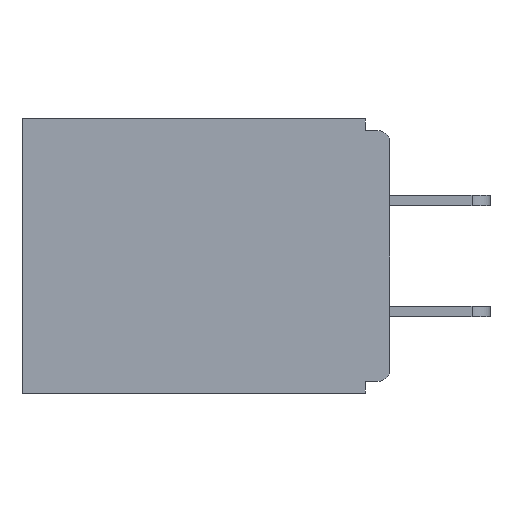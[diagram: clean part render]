
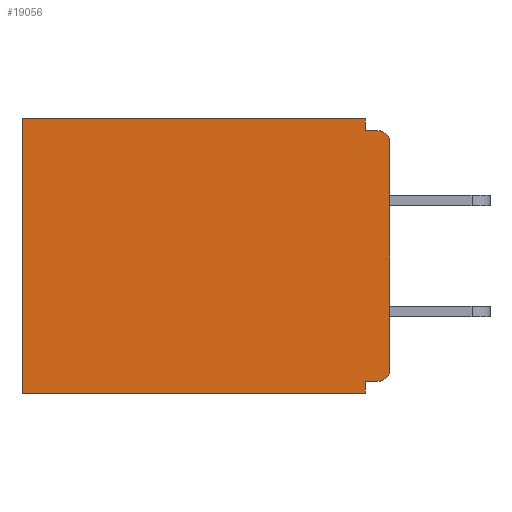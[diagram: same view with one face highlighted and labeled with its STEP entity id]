
A CAD part, left-side view. The second image highlights one B-rep face of the part: STEP entity #19056.
In plain terms, the highlighted planar face has unit normal (-1, 0, 0).
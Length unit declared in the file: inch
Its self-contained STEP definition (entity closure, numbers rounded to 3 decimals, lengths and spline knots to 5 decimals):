
#458 = VECTOR ( 'NONE', #2882, 39.37008 ) ;
#523 = VECTOR ( 'NONE', #17826, 39.37008 ) ;
#527 = CARTESIAN_POINT ( 'NONE',  ( 0.298, 0.031, -0.328 ) ) ;
#785 = DIRECTION ( 'NONE',  ( 0., 0., -1. ) ) ;
#814 = EDGE_CURVE ( 'NONE', #2526, #11283, #3351, .T. ) ;
#2526 = VERTEX_POINT ( 'NONE', #527 ) ;
#2698 = FACE_OUTER_BOUND ( 'NONE', #19223, .T. ) ;
#2882 = DIRECTION ( 'NONE',  ( 0., -1., 0. ) ) ;
#2897 = VERTEX_POINT ( 'NONE', #4062 ) ;
#3351 = LINE ( 'NONE', #8319, #10182 ) ;
#3595 = CARTESIAN_POINT ( 'NONE',  ( 0.298, 0.031, 0. ) ) ;
#3822 = VECTOR ( 'NONE', #15586, 39.37008 ) ;
#4062 = CARTESIAN_POINT ( 'NONE',  ( 0.298, 0., -0.03 ) ) ;
#4169 = CIRCLE ( 'NONE', #15703, 0.015 ) ;
#4626 = ORIENTED_EDGE ( 'NONE', *, *, #13898, .F. ) ;
#4696 = EDGE_CURVE ( 'NONE', #18968, #10914, #6065, .T. ) ;
#5461 = ORIENTED_EDGE ( 'NONE', *, *, #7891, .T. ) ;
#5559 = VERTEX_POINT ( 'NONE', #14626 ) ;
#6065 = LINE ( 'NONE', #19047, #458 ) ;
#6406 = CARTESIAN_POINT ( 'NONE',  ( 0.298, 0., -0.313 ) ) ;
#6590 = PLANE ( 'NONE',  #20074 ) ;
#7225 = CARTESIAN_POINT ( 'NONE',  ( 0.298, 0.015, -0.313 ) ) ;
#7318 = EDGE_CURVE ( 'NONE', #2897, #11034, #8191, .T. ) ;
#7408 = ORIENTED_EDGE ( 'NONE', *, *, #19416, .T. ) ;
#7878 = LINE ( 'NONE', #16179, #523 ) ;
#7891 = EDGE_CURVE ( 'NONE', #2897, #10914, #4169, .T. ) ;
#8170 = DIRECTION ( 'NONE',  ( 0., 1., 0. ) ) ;
#8191 = LINE ( 'NONE', #14476, #10974 ) ;
#8195 = DIRECTION ( 'NONE',  ( 1., 0., 0. ) ) ;
#8257 = CARTESIAN_POINT ( 'NONE',  ( 0.298, 0.031, -0.015 ) ) ;
#8319 = CARTESIAN_POINT ( 'NONE',  ( 0.298, 0.031, -0.343 ) ) ;
#8585 = VERTEX_POINT ( 'NONE', #10213 ) ;
#9103 = CARTESIAN_POINT ( 'NONE',  ( 0.298, 0.031, -0.343 ) ) ;
#10182 = VECTOR ( 'NONE', #19724, 39.37008 ) ;
#10213 = CARTESIAN_POINT ( 'NONE',  ( 0.298, 0.46, 0. ) ) ;
#10231 = ORIENTED_EDGE ( 'NONE', *, *, #7318, .F. ) ;
#10466 = DIRECTION ( 'NONE',  ( -1., 0., 0. ) ) ;
#10502 = VECTOR ( 'NONE', #12996, 39.37008 ) ;
#10834 = CARTESIAN_POINT ( 'NONE',  ( 0.298, 0.015, -0.015 ) ) ;
#10914 = VERTEX_POINT ( 'NONE', #10834 ) ;
#10974 = VECTOR ( 'NONE', #19474, 39.37008 ) ;
#11034 = VERTEX_POINT ( 'NONE', #6406 ) ;
#11144 = CARTESIAN_POINT ( 'NONE',  ( 0.298, 0.015, -0.03 ) ) ;
#11271 = LINE ( 'NONE', #20958, #10502 ) ;
#11283 = VERTEX_POINT ( 'NONE', #9103 ) ;
#11580 = ORIENTED_EDGE ( 'NONE', *, *, #14292, .T. ) ;
#12996 = DIRECTION ( 'NONE',  ( 0., 0., -1. ) ) ;
#13507 = ORIENTED_EDGE ( 'NONE', *, *, #814, .F. ) ;
#13559 = ORIENTED_EDGE ( 'NONE', *, *, #19782, .T. ) ;
#13715 = ORIENTED_EDGE ( 'NONE', *, *, #19529, .F. ) ;
#13898 = EDGE_CURVE ( 'NONE', #20474, #2526, #7878, .T. ) ;
#14291 = DIRECTION ( 'NONE',  ( 0., 0., -1. ) ) ;
#14292 = EDGE_CURVE ( 'NONE', #18573, #8585, #18849, .T. ) ;
#14476 = CARTESIAN_POINT ( 'NONE',  ( 0.298, 0., 0. ) ) ;
#14487 = CARTESIAN_POINT ( 'NONE',  ( 0.298, 0.015, -0.328 ) ) ;
#14626 = CARTESIAN_POINT ( 'NONE',  ( 0.298, 0.46, -0.343 ) ) ;
#15138 = CIRCLE ( 'NONE', #17802, 0.015 ) ;
#15299 = EDGE_CURVE ( 'NONE', #18573, #18968, #16001, .T. ) ;
#15586 = DIRECTION ( 'NONE',  ( 0., 1., 0. ) ) ;
#15703 = AXIS2_PLACEMENT_3D ( 'NONE', #11144, #20967, #14291 ) ;
#15724 = CARTESIAN_POINT ( 'NONE',  ( 0.298, 0., 0. ) ) ;
#16001 = LINE ( 'NONE', #19259, #18802 ) ;
#16046 = DIRECTION ( 'NONE',  ( 0., 0., -1. ) ) ;
#16179 = CARTESIAN_POINT ( 'NONE',  ( 0.298, 0., -0.328 ) ) ;
#16672 = VECTOR ( 'NONE', #8170, 39.37008 ) ;
#17802 = AXIS2_PLACEMENT_3D ( 'NONE', #7225, #10466, #785 ) ;
#17826 = DIRECTION ( 'NONE',  ( 0., 1., 0. ) ) ;
#17959 = CARTESIAN_POINT ( 'NONE',  ( 0.298, 0., -0.343 ) ) ;
#17983 = CARTESIAN_POINT ( 'NONE',  ( 0.298, 0., 0. ) ) ;
#18557 = ORIENTED_EDGE ( 'NONE', *, *, #15299, .F. ) ;
#18573 = VERTEX_POINT ( 'NONE', #3595 ) ;
#18802 = VECTOR ( 'NONE', #16046, 39.37008 ) ;
#18849 = LINE ( 'NONE', #15724, #3822 ) ;
#18968 = VERTEX_POINT ( 'NONE', #8257 ) ;
#19047 = CARTESIAN_POINT ( 'NONE',  ( 0.298, 0., -0.015 ) ) ;
#19056 = ADVANCED_FACE ( 'NONE', ( #2698 ), #6590, .F. ) ;
#19223 = EDGE_LOOP ( 'NONE', ( #5461, #19794, #18557, #11580, #13559, #13715, #13507, #4626, #7408, #10231 ) ) ;
#19259 = CARTESIAN_POINT ( 'NONE',  ( 0.298, 0.031, -0.343 ) ) ;
#19416 = EDGE_CURVE ( 'NONE', #20474, #11034, #15138, .T. ) ;
#19474 = DIRECTION ( 'NONE',  ( 0., 0., -1. ) ) ;
#19529 = EDGE_CURVE ( 'NONE', #11283, #5559, #20972, .T. ) ;
#19608 = DIRECTION ( 'NONE',  ( 0., 0., -1. ) ) ;
#19724 = DIRECTION ( 'NONE',  ( 0., 0., -1. ) ) ;
#19782 = EDGE_CURVE ( 'NONE', #8585, #5559, #11271, .T. ) ;
#19794 = ORIENTED_EDGE ( 'NONE', *, *, #4696, .F. ) ;
#20074 = AXIS2_PLACEMENT_3D ( 'NONE', #17983, #8195, #19608 ) ;
#20474 = VERTEX_POINT ( 'NONE', #14487 ) ;
#20958 = CARTESIAN_POINT ( 'NONE',  ( 0.298, 0.46, 0. ) ) ;
#20967 = DIRECTION ( 'NONE',  ( -1., 0., 0. ) ) ;
#20972 = LINE ( 'NONE', #17959, #16672 ) ;
